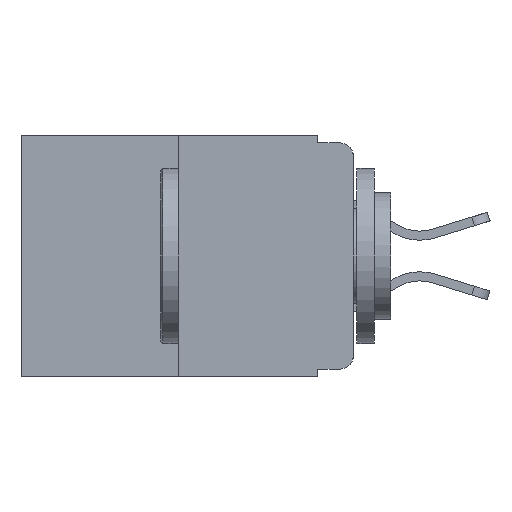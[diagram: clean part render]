
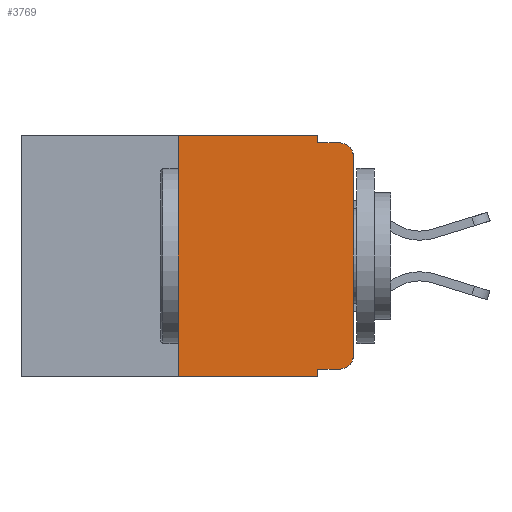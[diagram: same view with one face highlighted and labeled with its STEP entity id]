
A CAD part, left-side view. The second image highlights one B-rep face of the part: STEP entity #3769.
In plain terms, the highlighted planar face has unit normal (-1, 0, 0).
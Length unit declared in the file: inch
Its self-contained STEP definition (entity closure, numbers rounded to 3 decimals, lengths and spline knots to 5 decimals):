
#12 = EDGE_CURVE ( 'NONE', #6642, #11622, #4981, .T. ) ;
#313 = ORIENTED_EDGE ( 'NONE', *, *, #12583, .F. ) ;
#432 = CIRCLE ( 'NONE', #17550, 0.02 ) ;
#628 = ORIENTED_EDGE ( 'NONE', *, *, #8646, .T. ) ;
#661 = VECTOR ( 'NONE', #11392, 39.37008 ) ;
#1013 = CARTESIAN_POINT ( 'NONE',  ( 0., 0.473, 0. ) ) ;
#1023 = ORIENTED_EDGE ( 'NONE', *, *, #18720, .F. ) ;
#1383 = CARTESIAN_POINT ( 'NONE',  ( 0., 0.051, -0.01 ) ) ;
#2138 = CARTESIAN_POINT ( 'NONE',  ( 0., 0., 0. ) ) ;
#2233 = VERTEX_POINT ( 'NONE', #8394 ) ;
#2603 = DIRECTION ( 'NONE',  ( 0., 0., -1. ) ) ;
#2654 = ORIENTED_EDGE ( 'NONE', *, *, #12221, .T. ) ;
#2844 = CIRCLE ( 'NONE', #6924, 0.02 ) ;
#2866 = CARTESIAN_POINT ( 'NONE',  ( 0., 0.473, -0.343 ) ) ;
#2885 = ORIENTED_EDGE ( 'NONE', *, *, #4246, .T. ) ;
#3203 = DIRECTION ( 'NONE',  ( 0., -1., 0. ) ) ;
#3250 = CARTESIAN_POINT ( 'NONE',  ( 0., 0.051, 0. ) ) ;
#3310 = CARTESIAN_POINT ( 'NONE',  ( 0., 0.02, -0.03 ) ) ;
#3411 = LINE ( 'NONE', #2138, #19459 ) ;
#3426 = EDGE_LOOP ( 'NONE', ( #4017, #2654, #313, #10356, #3458, #10792, #12756, #1023, #2885, #628 ) ) ;
#3458 = ORIENTED_EDGE ( 'NONE', *, *, #10007, .F. ) ;
#3634 = CARTESIAN_POINT ( 'NONE',  ( 0., 0.25, 0. ) ) ;
#3769 = ADVANCED_FACE ( 'NONE', ( #5468 ), #17010, .F. ) ;
#4017 = ORIENTED_EDGE ( 'NONE', *, *, #13191, .T. ) ;
#4246 = EDGE_CURVE ( 'NONE', #6170, #19439, #8605, .T. ) ;
#4368 = LINE ( 'NONE', #3634, #11614 ) ;
#4375 = VERTEX_POINT ( 'NONE', #11376 ) ;
#4570 = LINE ( 'NONE', #3250, #13650 ) ;
#4893 = DIRECTION ( 'NONE',  ( 0., 0., -1. ) ) ;
#4981 = LINE ( 'NONE', #2866, #8620 ) ;
#5092 = AXIS2_PLACEMENT_3D ( 'NONE', #1013, #8476, #2603 ) ;
#5468 = FACE_OUTER_BOUND ( 'NONE', #3426, .T. ) ;
#6062 = CARTESIAN_POINT ( 'NONE',  ( 0., 0.02, -0.333 ) ) ;
#6170 = VERTEX_POINT ( 'NONE', #6746 ) ;
#6288 = CARTESIAN_POINT ( 'NONE',  ( 0., 0.25, 0. ) ) ;
#6642 = VERTEX_POINT ( 'NONE', #18295 ) ;
#6746 = CARTESIAN_POINT ( 'NONE',  ( 0., 0.051, -0.333 ) ) ;
#6924 = AXIS2_PLACEMENT_3D ( 'NONE', #18142, #9253, #19602 ) ;
#7649 = EDGE_CURVE ( 'NONE', #6642, #12715, #4368, .T. ) ;
#8309 = DIRECTION ( 'NONE',  ( 0., 0., 1. ) ) ;
#8394 = CARTESIAN_POINT ( 'NONE',  ( 0., 0., -0.03 ) ) ;
#8476 = DIRECTION ( 'NONE',  ( 1., 0., 0. ) ) ;
#8605 = LINE ( 'NONE', #16582, #9094 ) ;
#8620 = VECTOR ( 'NONE', #9485, 39.37008 ) ;
#8646 = EDGE_CURVE ( 'NONE', #19439, #13374, #2844, .T. ) ;
#8759 = EDGE_CURVE ( 'NONE', #16936, #4375, #4570, .T. ) ;
#9094 = VECTOR ( 'NONE', #9358, 39.37008 ) ;
#9253 = DIRECTION ( 'NONE',  ( -1., 0., 0. ) ) ;
#9358 = DIRECTION ( 'NONE',  ( 0., -1., 0. ) ) ;
#9485 = DIRECTION ( 'NONE',  ( 0., -1., 0. ) ) ;
#9857 = CARTESIAN_POINT ( 'NONE',  ( 0., 0.051, 0. ) ) ;
#10007 = EDGE_CURVE ( 'NONE', #12715, #16936, #18414, .T. ) ;
#10356 = ORIENTED_EDGE ( 'NONE', *, *, #8759, .F. ) ;
#10792 = ORIENTED_EDGE ( 'NONE', *, *, #7649, .F. ) ;
#11007 = DIRECTION ( 'NONE',  ( 0., 0., -1. ) ) ;
#11376 = CARTESIAN_POINT ( 'NONE',  ( 0., 0.051, -0.01 ) ) ;
#11392 = DIRECTION ( 'NONE',  ( 0., 0., -1. ) ) ;
#11449 = DIRECTION ( 'NONE',  ( 0., 0., 1. ) ) ;
#11614 = VECTOR ( 'NONE', #8309, 39.37008 ) ;
#11622 = VERTEX_POINT ( 'NONE', #18464 ) ;
#11646 = CARTESIAN_POINT ( 'NONE',  ( 0., 0.051, 0. ) ) ;
#12221 = EDGE_CURVE ( 'NONE', #2233, #15175, #432, .T. ) ;
#12448 = CARTESIAN_POINT ( 'NONE',  ( 0., 0.473, 0. ) ) ;
#12583 = EDGE_CURVE ( 'NONE', #4375, #15175, #18346, .T. ) ;
#12715 = VERTEX_POINT ( 'NONE', #6288 ) ;
#12756 = ORIENTED_EDGE ( 'NONE', *, *, #12, .T. ) ;
#13014 = LINE ( 'NONE', #9857, #661 ) ;
#13191 = EDGE_CURVE ( 'NONE', #13374, #2233, #3411, .T. ) ;
#13374 = VERTEX_POINT ( 'NONE', #14706 ) ;
#13650 = VECTOR ( 'NONE', #11007, 39.37008 ) ;
#14035 = DIRECTION ( 'NONE',  ( -1., 0., 0. ) ) ;
#14445 = VECTOR ( 'NONE', #16658, 39.37008 ) ;
#14515 = VECTOR ( 'NONE', #3203, 39.37008 ) ;
#14706 = CARTESIAN_POINT ( 'NONE',  ( 0., 0., -0.313 ) ) ;
#15175 = VERTEX_POINT ( 'NONE', #19033 ) ;
#16582 = CARTESIAN_POINT ( 'NONE',  ( 0., 0.051, -0.333 ) ) ;
#16658 = DIRECTION ( 'NONE',  ( 0., -1., 0. ) ) ;
#16936 = VERTEX_POINT ( 'NONE', #11646 ) ;
#17010 = PLANE ( 'NONE',  #5092 ) ;
#17550 = AXIS2_PLACEMENT_3D ( 'NONE', #3310, #14035, #4893 ) ;
#18142 = CARTESIAN_POINT ( 'NONE',  ( 0., 0.02, -0.313 ) ) ;
#18295 = CARTESIAN_POINT ( 'NONE',  ( 0., 0.25, -0.343 ) ) ;
#18346 = LINE ( 'NONE', #1383, #14445 ) ;
#18414 = LINE ( 'NONE', #12448, #14515 ) ;
#18464 = CARTESIAN_POINT ( 'NONE',  ( 0., 0.051, -0.343 ) ) ;
#18720 = EDGE_CURVE ( 'NONE', #6170, #11622, #13014, .T. ) ;
#19033 = CARTESIAN_POINT ( 'NONE',  ( 0., 0.02, -0.01 ) ) ;
#19439 = VERTEX_POINT ( 'NONE', #6062 ) ;
#19459 = VECTOR ( 'NONE', #11449, 39.37008 ) ;
#19602 = DIRECTION ( 'NONE',  ( 0., 0., -1. ) ) ;
